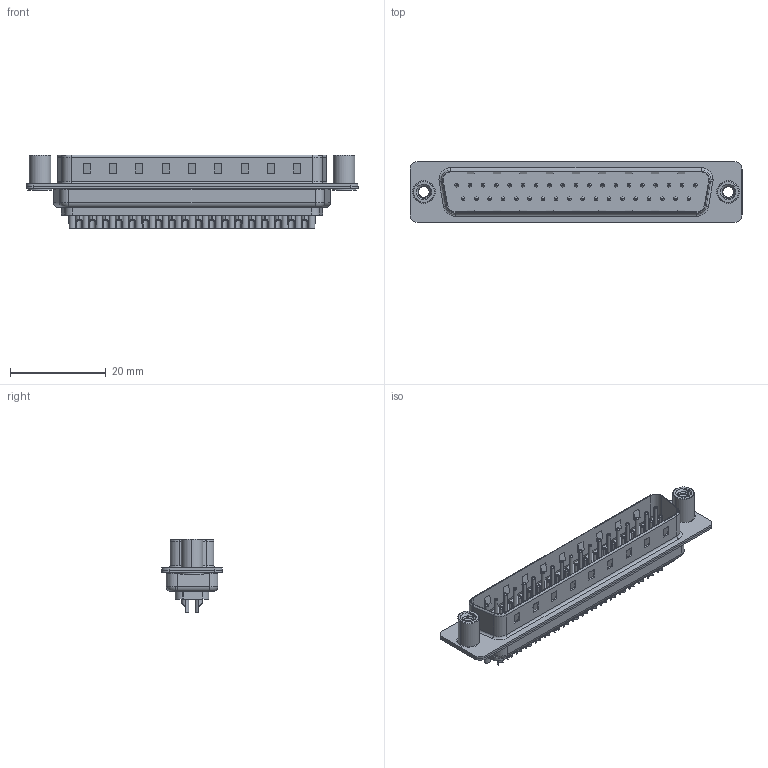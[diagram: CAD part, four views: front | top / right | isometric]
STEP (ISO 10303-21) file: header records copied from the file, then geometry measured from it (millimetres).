
FILE_DESCRIPTION (( 'STEP AP203' ), '1' );
FILE_NAME ('627-037-222-248.STEP', '2020-07-15T02:24:53', ( '' ), ( '' ), 'SwSTEP 2.0', 'SolidWorks 2020', '' );
FILE_SCHEMA (( 'CONFIG_CONTROL_DESIGN' ));
Length unit declared in the file: millimetre
Products named in the file (7): 627 Housing_37 LP; 627 Shell Rear_37 Contacts; 627 Contact Row 1_22L; 627 Contact Row 2_22L; 627-037-222-248; 627 Shell Front_37 Contacts; 627 4-40 Threaded Standoff
Assembly tree (42 placements, depth 2):
  627-037-222-248
    627 Housing_37 LP
    627 Shell Front_37 Contacts
    627 Shell Rear_37 Contacts
    627 Contact Row 1_22L  x19
    627 Contact Row 2_22L  x18
    627 4-40 Threaded Standoff  x2
Bounding box: 69.3 x 12.6 x 15.35 mm (x, y, z)
Volume: 3777.5 mm3; surface area: 10951.8 mm2
Topology: 42 solids, 42 shells, 2814 faces, 7217 edges, 4574 vertices
Faces by surface type: cylinder 1242, torus 827, plane 723, cone 16, bspline 6
Entity records: 27737 total; most frequent: CARTESIAN_POINT 6004, DIRECTION 4492, ORIENTED_EDGE 3960, EDGE_CURVE 1980, AXIS2_PLACEMENT_3D 1761, VERTEX_POINT 1272, EDGE_LOOP 1012, VECTOR 970
